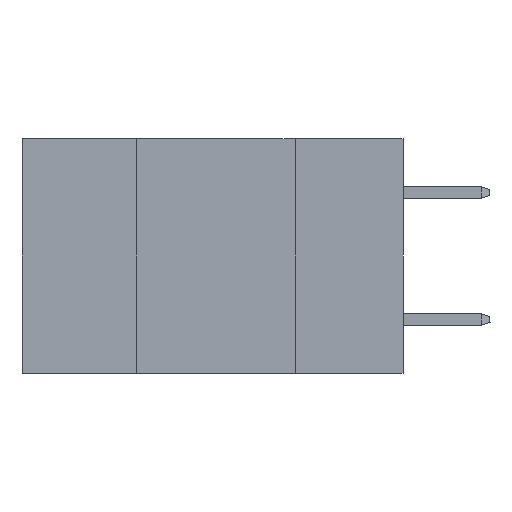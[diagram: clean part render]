
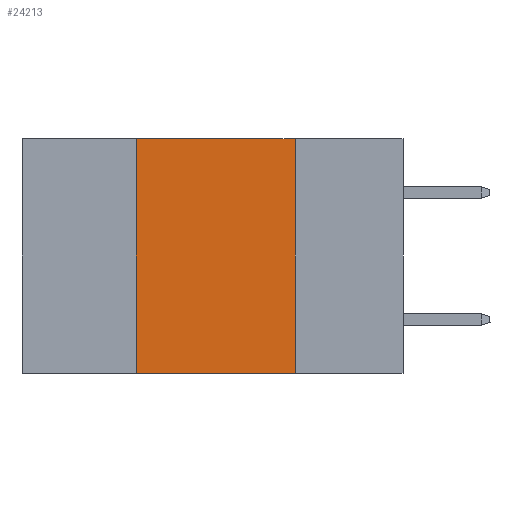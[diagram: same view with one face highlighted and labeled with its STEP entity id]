
A CAD part, left-side view. The second image highlights one B-rep face of the part: STEP entity #24213.
In plain terms, the highlighted planar face has unit normal (-1, 0, 0).
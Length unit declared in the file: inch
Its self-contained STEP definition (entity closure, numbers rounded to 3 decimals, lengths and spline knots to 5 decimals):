
#505 = DIRECTION ( 'NONE',  ( 0., 0., 1. ) ) ;
#2732 = EDGE_CURVE ( 'NONE', #21608, #3737, #7728, .T. ) ;
#2806 = VERTEX_POINT ( 'NONE', #14282 ) ;
#2969 = EDGE_CURVE ( 'NONE', #2806, #3737, #21164, .T. ) ;
#3737 = VERTEX_POINT ( 'NONE', #15650 ) ;
#3860 = CARTESIAN_POINT ( 'NONE',  ( 0., 0.6, -0.37 ) ) ;
#5582 = VECTOR ( 'NONE', #24954, 39.37008 ) ;
#5654 = CARTESIAN_POINT ( 'NONE',  ( 0., 0.17, 0. ) ) ;
#5800 = DIRECTION ( 'NONE',  ( 0., 0., -1. ) ) ;
#6005 = EDGE_LOOP ( 'NONE', ( #19282, #14936, #24323, #17566 ) ) ;
#6473 = DIRECTION ( 'NONE',  ( 1., 0., 0. ) ) ;
#7162 = AXIS2_PLACEMENT_3D ( 'NONE', #10057, #6473, #23899 ) ;
#7258 = LINE ( 'NONE', #16813, #5582 ) ;
#7581 = VECTOR ( 'NONE', #5800, 39.37008 ) ;
#7728 = LINE ( 'NONE', #23370, #7581 ) ;
#10057 = CARTESIAN_POINT ( 'NONE',  ( 0., 0.6, 0. ) ) ;
#10218 = LINE ( 'NONE', #18055, #15027 ) ;
#11653 = DIRECTION ( 'NONE',  ( 0., -1., 0. ) ) ;
#14116 = EDGE_CURVE ( 'NONE', #16357, #21608, #7258, .T. ) ;
#14282 = CARTESIAN_POINT ( 'NONE',  ( 0., 0.42, -0.37 ) ) ;
#14447 = PLANE ( 'NONE',  #7162 ) ;
#14936 = ORIENTED_EDGE ( 'NONE', *, *, #14116, .F. ) ;
#15027 = VECTOR ( 'NONE', #505, 39.37008 ) ;
#15650 = CARTESIAN_POINT ( 'NONE',  ( 0., 0.17, -0.37 ) ) ;
#15995 = FACE_OUTER_BOUND ( 'NONE', #6005, .T. ) ;
#16357 = VERTEX_POINT ( 'NONE', #21290 ) ;
#16813 = CARTESIAN_POINT ( 'NONE',  ( 0., 0.6, 0. ) ) ;
#17566 = ORIENTED_EDGE ( 'NONE', *, *, #2969, .T. ) ;
#18055 = CARTESIAN_POINT ( 'NONE',  ( 0., 0.42, 0. ) ) ;
#19282 = ORIENTED_EDGE ( 'NONE', *, *, #2732, .F. ) ;
#21092 = VECTOR ( 'NONE', #11653, 39.37008 ) ;
#21164 = LINE ( 'NONE', #3860, #21092 ) ;
#21290 = CARTESIAN_POINT ( 'NONE',  ( 0., 0.42, 0. ) ) ;
#21608 = VERTEX_POINT ( 'NONE', #5654 ) ;
#23370 = CARTESIAN_POINT ( 'NONE',  ( 0., 0.17, 0. ) ) ;
#23695 = EDGE_CURVE ( 'NONE', #2806, #16357, #10218, .T. ) ;
#23899 = DIRECTION ( 'NONE',  ( 0., 0., -1. ) ) ;
#24213 = ADVANCED_FACE ( 'NONE', ( #15995 ), #14447, .F. ) ;
#24323 = ORIENTED_EDGE ( 'NONE', *, *, #23695, .F. ) ;
#24954 = DIRECTION ( 'NONE',  ( 0., -1., 0. ) ) ;
